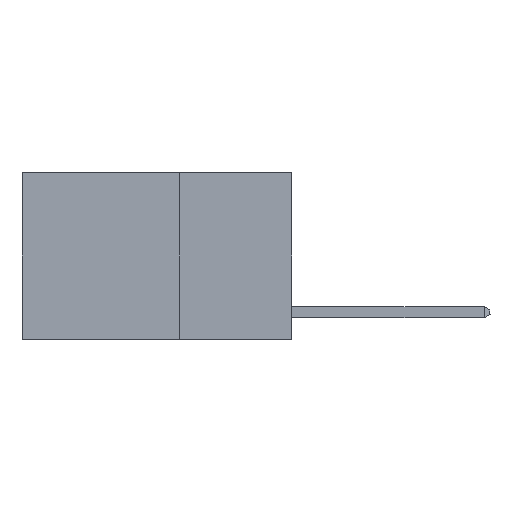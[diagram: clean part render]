
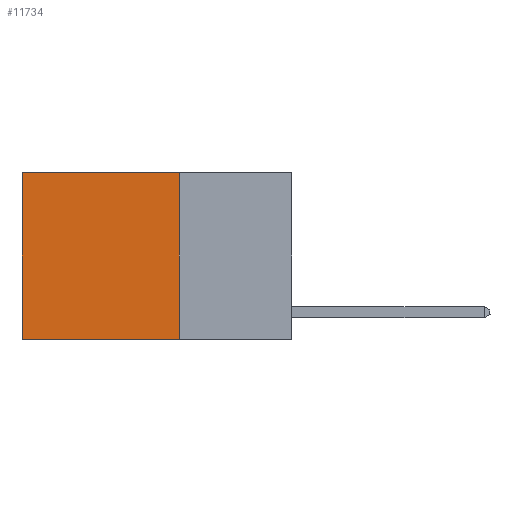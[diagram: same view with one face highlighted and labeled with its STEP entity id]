
A CAD part, left-side view. The second image highlights one B-rep face of the part: STEP entity #11734.
In plain terms, the highlighted planar face has unit normal (-1, 0, 0).
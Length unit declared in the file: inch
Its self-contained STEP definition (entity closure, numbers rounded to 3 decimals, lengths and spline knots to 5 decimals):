
#219 = VERTEX_POINT ( 'NONE', #7886 ) ;
#409 = CARTESIAN_POINT ( 'NONE',  ( 0.2625, 0.6, 0. ) ) ;
#861 = LINE ( 'NONE', #959, #2926 ) ;
#959 = CARTESIAN_POINT ( 'NONE',  ( 0.2625, 0.25, 0. ) ) ;
#1282 = ORIENTED_EDGE ( 'NONE', *, *, #5134, .T. ) ;
#1320 = CARTESIAN_POINT ( 'NONE',  ( 0.2625, 0.25, 0. ) ) ;
#1616 = PLANE ( 'NONE',  #18488 ) ;
#1846 = ORIENTED_EDGE ( 'NONE', *, *, #20395, .T. ) ;
#2832 = VERTEX_POINT ( 'NONE', #18605 ) ;
#2926 = VECTOR ( 'NONE', #10930, 39.37008 ) ;
#3352 = DIRECTION ( 'NONE',  ( 0., 0., -1. ) ) ;
#4266 = CARTESIAN_POINT ( 'NONE',  ( 0.2625, 0.6, 0. ) ) ;
#5134 = EDGE_CURVE ( 'NONE', #14244, #19135, #861, .T. ) ;
#5213 = VECTOR ( 'NONE', #14766, 39.37008 ) ;
#6178 = ORIENTED_EDGE ( 'NONE', *, *, #18082, .F. ) ;
#7508 = DIRECTION ( 'NONE',  ( 0., 0., -1. ) ) ;
#7886 = CARTESIAN_POINT ( 'NONE',  ( 0.2625, 0.25, -0.37 ) ) ;
#8855 = EDGE_CURVE ( 'NONE', #219, #2832, #10170, .T. ) ;
#10170 = LINE ( 'NONE', #11904, #21160 ) ;
#10930 = DIRECTION ( 'NONE',  ( 0., 1., 0. ) ) ;
#11734 = ADVANCED_FACE ( 'NONE', ( #13427 ), #1616, .F. ) ;
#11904 = CARTESIAN_POINT ( 'NONE',  ( 0.2625, 0.25, -0.37 ) ) ;
#12101 = DIRECTION ( 'NONE',  ( 0., 1., 0. ) ) ;
#13283 = ORIENTED_EDGE ( 'NONE', *, *, #8855, .F. ) ;
#13427 = FACE_OUTER_BOUND ( 'NONE', #13460, .T. ) ;
#13460 = EDGE_LOOP ( 'NONE', ( #1846, #13283, #6178, #1282 ) ) ;
#14244 = VERTEX_POINT ( 'NONE', #15967 ) ;
#14766 = DIRECTION ( 'NONE',  ( 0., 0., -1. ) ) ;
#15967 = CARTESIAN_POINT ( 'NONE',  ( 0.2625, 0.25, 0. ) ) ;
#16374 = DIRECTION ( 'NONE',  ( 1., 0., 0. ) ) ;
#17690 = VECTOR ( 'NONE', #7508, 39.37008 ) ;
#18082 = EDGE_CURVE ( 'NONE', #14244, #219, #19139, .T. ) ;
#18488 = AXIS2_PLACEMENT_3D ( 'NONE', #19964, #16374, #3352 ) ;
#18605 = CARTESIAN_POINT ( 'NONE',  ( 0.2625, 0.6, -0.37 ) ) ;
#19132 = LINE ( 'NONE', #4266, #5213 ) ;
#19135 = VERTEX_POINT ( 'NONE', #409 ) ;
#19139 = LINE ( 'NONE', #1320, #17690 ) ;
#19964 = CARTESIAN_POINT ( 'NONE',  ( 0.2625, 0.25, 0. ) ) ;
#20395 = EDGE_CURVE ( 'NONE', #19135, #2832, #19132, .T. ) ;
#21160 = VECTOR ( 'NONE', #12101, 39.37008 ) ;
